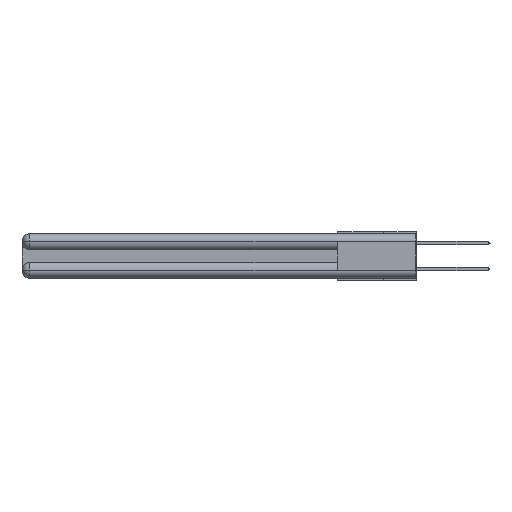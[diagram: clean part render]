
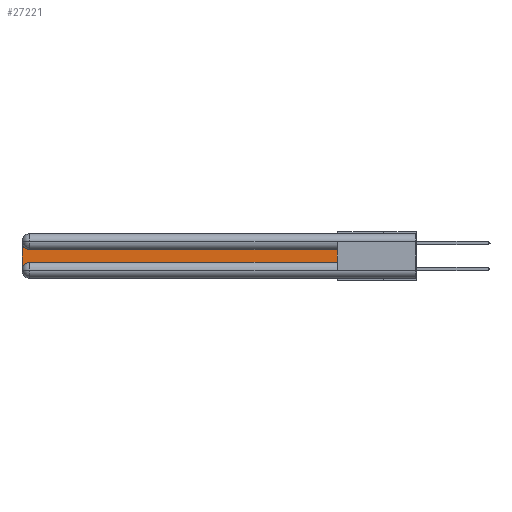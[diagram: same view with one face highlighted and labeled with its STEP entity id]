
A CAD part, left-side view. The second image highlights one B-rep face of the part: STEP entity #27221.
In plain terms, the highlighted planar face has unit normal (-1, 0, 0).
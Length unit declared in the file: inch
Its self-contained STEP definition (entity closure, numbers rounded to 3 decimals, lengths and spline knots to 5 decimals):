
#234 = FACE_OUTER_BOUND ( 'NONE', #31563, .T. ) ;
#878 = EDGE_CURVE ( 'NONE', #11589, #2956, #18227, .T. ) ;
#901 = VERTEX_POINT ( 'NONE', #11097 ) ;
#1298 = CARTESIAN_POINT ( 'NONE',  ( 0.075, 3., -0.2175 ) ) ;
#2956 = VERTEX_POINT ( 'NONE', #11110 ) ;
#3972 = DIRECTION ( 'NONE',  ( 0., 0., -1. ) ) ;
#4734 = PLANE ( 'NONE',  #5922 ) ;
#5922 = AXIS2_PLACEMENT_3D ( 'NONE', #24779, #17527, #14815 ) ;
#6085 = CARTESIAN_POINT ( 'NONE',  ( 0.075, 0.6, -0.2175 ) ) ;
#7162 = VECTOR ( 'NONE', #32312, 39.37008 ) ;
#7714 = DIRECTION ( 'NONE',  ( 0., 0., -1. ) ) ;
#7885 = EDGE_CURVE ( 'NONE', #11298, #11407, #14054, .T. ) ;
#8617 = ORIENTED_EDGE ( 'NONE', *, *, #8688, .T. ) ;
#8688 = EDGE_CURVE ( 'NONE', #2956, #11298, #21631, .T. ) ;
#11097 = CARTESIAN_POINT ( 'NONE',  ( 0.075, 0.6, -0.2175 ) ) ;
#11110 = CARTESIAN_POINT ( 'NONE',  ( 0.075, 2.94, -0.1225 ) ) ;
#11298 = VERTEX_POINT ( 'NONE', #21775 ) ;
#11407 = VERTEX_POINT ( 'NONE', #14888 ) ;
#11457 = VECTOR ( 'NONE', #30943, 39.37008 ) ;
#11589 = VERTEX_POINT ( 'NONE', #13522 ) ;
#12473 = DIRECTION ( 'NONE',  ( 1., 0., 0. ) ) ;
#12668 = AXIS2_PLACEMENT_3D ( 'NONE', #20332, #12473, #7714 ) ;
#12994 = CARTESIAN_POINT ( 'NONE',  ( 0.075, 0.6, -0.1225 ) ) ;
#13198 = AXIS2_PLACEMENT_3D ( 'NONE', #16246, #21617, #23626 ) ;
#13522 = CARTESIAN_POINT ( 'NONE',  ( 0.075, 0.6, -0.1225 ) ) ;
#13706 = ORIENTED_EDGE ( 'NONE', *, *, #878, .T. ) ;
#14054 = LINE ( 'NONE', #1298, #26479 ) ;
#14370 = CARTESIAN_POINT ( 'NONE',  ( 0.075, 0.6, -0.2175 ) ) ;
#14497 = EDGE_CURVE ( 'NONE', #11407, #28088, #27352, .T. ) ;
#14815 = DIRECTION ( 'NONE',  ( 0., 0., -1. ) ) ;
#14888 = CARTESIAN_POINT ( 'NONE',  ( 0.075, 3., -0.2775 ) ) ;
#16246 = CARTESIAN_POINT ( 'NONE',  ( 0.075, 2.94, -0.0625 ) ) ;
#17527 = DIRECTION ( 'NONE',  ( 1., 0., 0. ) ) ;
#18227 = LINE ( 'NONE', #12994, #11457 ) ;
#18803 = ORIENTED_EDGE ( 'NONE', *, *, #14497, .T. ) ;
#20332 = CARTESIAN_POINT ( 'NONE',  ( 0.075, 2.94, -0.2775 ) ) ;
#20898 = LINE ( 'NONE', #14370, #7162 ) ;
#21617 = DIRECTION ( 'NONE',  ( 1., 0., 0. ) ) ;
#21631 = CIRCLE ( 'NONE', #13198, 0.06 ) ;
#21775 = CARTESIAN_POINT ( 'NONE',  ( 0.075, 3., -0.0625 ) ) ;
#21856 = DIRECTION ( 'NONE',  ( 0., -1., 0. ) ) ;
#23626 = DIRECTION ( 'NONE',  ( 0., 0., -1. ) ) ;
#24779 = CARTESIAN_POINT ( 'NONE',  ( 0.075, 3., -0.1225 ) ) ;
#25128 = ORIENTED_EDGE ( 'NONE', *, *, #7885, .T. ) ;
#25289 = EDGE_CURVE ( 'NONE', #901, #11589, #20898, .T. ) ;
#25743 = EDGE_CURVE ( 'NONE', #28088, #901, #32100, .T. ) ;
#26479 = VECTOR ( 'NONE', #3972, 39.37008 ) ;
#27221 = ADVANCED_FACE ( 'NONE', ( #234 ), #4734, .F. ) ;
#27352 = CIRCLE ( 'NONE', #12668, 0.06 ) ;
#28088 = VERTEX_POINT ( 'NONE', #28929 ) ;
#28929 = CARTESIAN_POINT ( 'NONE',  ( 0.075, 2.94, -0.2175 ) ) ;
#30943 = DIRECTION ( 'NONE',  ( 0., 1., 0. ) ) ;
#31563 = EDGE_LOOP ( 'NONE', ( #13706, #8617, #25128, #18803, #33241, #31878 ) ) ;
#31878 = ORIENTED_EDGE ( 'NONE', *, *, #25289, .T. ) ;
#32100 = LINE ( 'NONE', #6085, #32893 ) ;
#32312 = DIRECTION ( 'NONE',  ( 0., 0., 1. ) ) ;
#32893 = VECTOR ( 'NONE', #21856, 39.37008 ) ;
#33241 = ORIENTED_EDGE ( 'NONE', *, *, #25743, .T. ) ;
